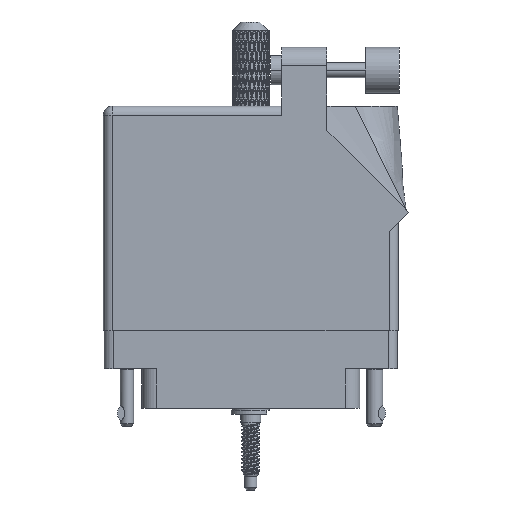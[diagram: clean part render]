
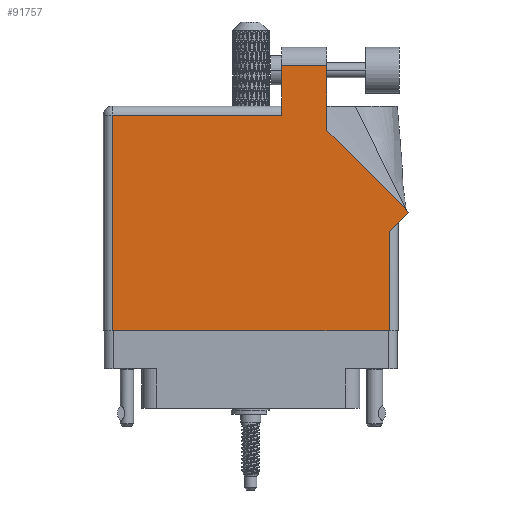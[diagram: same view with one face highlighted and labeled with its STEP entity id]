
A CAD part, front view. The second image highlights one B-rep face of the part: STEP entity #91757.
In plain terms, the highlighted face is planar.
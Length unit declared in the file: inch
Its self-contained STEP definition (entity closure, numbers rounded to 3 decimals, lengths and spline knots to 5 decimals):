
#317 = DIRECTION ( 'NONE',  ( 0., -1., 0. ) ) ;
#947 = EDGE_CURVE ( 'NONE', #90187, #91917, #111009, .T. ) ;
#8537 = EDGE_CURVE ( 'NONE', #61859, #90187, #59138, .T. ) ;
#8980 = CARTESIAN_POINT ( 'NONE',  ( 0.062, 0., 0. ) ) ;
#9737 = ORIENTED_EDGE ( 'NONE', *, *, #75229, .T. ) ;
#11830 = ORIENTED_EDGE ( 'NONE', *, *, #50496, .T. ) ;
#11861 = PLANE ( 'NONE',  #49592 ) ;
#12321 = VECTOR ( 'NONE', #55335, 39.37008 ) ;
#12627 = VERTEX_POINT ( 'NONE', #32997 ) ;
#14518 = VERTEX_POINT ( 'NONE', #90886 ) ;
#14753 = CARTESIAN_POINT ( 'NONE',  ( 0.062, 0., 0. ) ) ;
#14939 = LINE ( 'NONE', #14753, #58981 ) ;
#16707 = LINE ( 'NONE', #35002, #40089 ) ;
#18632 = CARTESIAN_POINT ( 'NONE',  ( 1.217, 1.468, 0. ) ) ;
#19074 = VECTOR ( 'NONE', #67660, 39.37008 ) ;
#23572 = DIRECTION ( 'NONE',  ( 0., -1., 0. ) ) ;
#23972 = VECTOR ( 'NONE', #54959, 39.37008 ) ;
#27790 = CARTESIAN_POINT ( 'NONE',  ( 1.524, 1.805, 0. ) ) ;
#28742 = CARTESIAN_POINT ( 'NONE',  ( 1.217, 1.805, 0. ) ) ;
#29762 = FACE_OUTER_BOUND ( 'NONE', #113261, .T. ) ;
#31919 = ORIENTED_EDGE ( 'NONE', *, *, #8537, .T. ) ;
#32997 = CARTESIAN_POINT ( 'NONE',  ( 0.062, 1.468, 0. ) ) ;
#35002 = CARTESIAN_POINT ( 'NONE',  ( 0., 1.468, 0. ) ) ;
#36541 = LINE ( 'NONE', #103699, #87453 ) ;
#40089 = VECTOR ( 'NONE', #51976, 39.37008 ) ;
#40138 = ORIENTED_EDGE ( 'NONE', *, *, #78033, .T. ) ;
#45243 = VECTOR ( 'NONE', #93027, 39.37008 ) ;
#45852 = VERTEX_POINT ( 'NONE', #95801 ) ;
#46694 = VERTEX_POINT ( 'NONE', #8980 ) ;
#47373 = LINE ( 'NONE', #89535, #23972 ) ;
#49592 = AXIS2_PLACEMENT_3D ( 'NONE', #72992, #64934, #90665 ) ;
#50496 = EDGE_CURVE ( 'NONE', #46694, #45852, #97709, .T. ) ;
#51976 = DIRECTION ( 'NONE',  ( -1., 0., 0. ) ) ;
#54249 = CARTESIAN_POINT ( 'NONE',  ( 1.217, 1.805, 0. ) ) ;
#54959 = DIRECTION ( 'NONE',  ( 0.707, 0.707, 0. ) ) ;
#55335 = DIRECTION ( 'NONE',  ( -1., 0., 0. ) ) ;
#58038 = CARTESIAN_POINT ( 'NONE',  ( 1.524, 1.36442, 0. ) ) ;
#58239 = ORIENTED_EDGE ( 'NONE', *, *, #58539, .T. ) ;
#58539 = EDGE_CURVE ( 'NONE', #80686, #61859, #89275, .T. ) ;
#58981 = VECTOR ( 'NONE', #23572, 39.37008 ) ;
#59138 = LINE ( 'NONE', #28742, #12321 ) ;
#61859 = VERTEX_POINT ( 'NONE', #27790 ) ;
#64934 = DIRECTION ( 'NONE',  ( 0., 0., -1. ) ) ;
#67660 = DIRECTION ( 'NONE',  ( 0., 1., 0. ) ) ;
#72992 = CARTESIAN_POINT ( 'NONE',  ( 0., 1.53, 0. ) ) ;
#74332 = VECTOR ( 'NONE', #102325, 39.37008 ) ;
#75229 = EDGE_CURVE ( 'NONE', #12627, #46694, #14939, .T. ) ;
#76223 = ORIENTED_EDGE ( 'NONE', *, *, #104407, .T. ) ;
#76444 = DIRECTION ( 'NONE',  ( -0.707, 0.707, 0. ) ) ;
#78033 = EDGE_CURVE ( 'NONE', #45852, #111731, #92173, .T. ) ;
#79378 = VECTOR ( 'NONE', #317, 39.37008 ) ;
#80686 = VERTEX_POINT ( 'NONE', #107710 ) ;
#85687 = CARTESIAN_POINT ( 'NONE',  ( 1.948, 0.737, 0. ) ) ;
#87453 = VECTOR ( 'NONE', #76444, 39.37008 ) ;
#89275 = LINE ( 'NONE', #58038, #19074 ) ;
#89535 = CARTESIAN_POINT ( 'NONE',  ( 2.01, 0.737, 0. ) ) ;
#90187 = VERTEX_POINT ( 'NONE', #54249 ) ;
#90665 = DIRECTION ( 'NONE',  ( -1., 0., 0. ) ) ;
#90886 = CARTESIAN_POINT ( 'NONE',  ( 2.08071, 0.80771, 0. ) ) ;
#91757 = ADVANCED_FACE ( 'NONE', ( #29762 ), #11861, .F. ) ;
#91917 = VERTEX_POINT ( 'NONE', #18632 ) ;
#92173 = LINE ( 'NONE', #85687, #45243 ) ;
#93027 = DIRECTION ( 'NONE',  ( 0., 1., 0. ) ) ;
#95260 = CARTESIAN_POINT ( 'NONE',  ( 1.948, 0.675, 0. ) ) ;
#95801 = CARTESIAN_POINT ( 'NONE',  ( 1.948, 0., 0. ) ) ;
#96772 = EDGE_CURVE ( 'NONE', #91917, #12627, #16707, .T. ) ;
#97709 = LINE ( 'NONE', #111520, #74332 ) ;
#97805 = ORIENTED_EDGE ( 'NONE', *, *, #102861, .T. ) ;
#102240 = ORIENTED_EDGE ( 'NONE', *, *, #96772, .T. ) ;
#102325 = DIRECTION ( 'NONE',  ( 1., 0., 0. ) ) ;
#102861 = EDGE_CURVE ( 'NONE', #14518, #80686, #36541, .T. ) ;
#103699 = CARTESIAN_POINT ( 'NONE',  ( 2.08071, 0.80771, 0. ) ) ;
#104407 = EDGE_CURVE ( 'NONE', #111731, #14518, #47373, .T. ) ;
#105663 = CARTESIAN_POINT ( 'NONE',  ( 1.217, 1.53, 0. ) ) ;
#107710 = CARTESIAN_POINT ( 'NONE',  ( 1.524, 1.36442, 0. ) ) ;
#111009 = LINE ( 'NONE', #105663, #79378 ) ;
#111520 = CARTESIAN_POINT ( 'NONE',  ( 0., 0., 0. ) ) ;
#111731 = VERTEX_POINT ( 'NONE', #95260 ) ;
#112389 = ORIENTED_EDGE ( 'NONE', *, *, #947, .T. ) ;
#113261 = EDGE_LOOP ( 'NONE', ( #58239, #31919, #112389, #102240, #9737, #11830, #40138, #76223, #97805 ) ) ;
